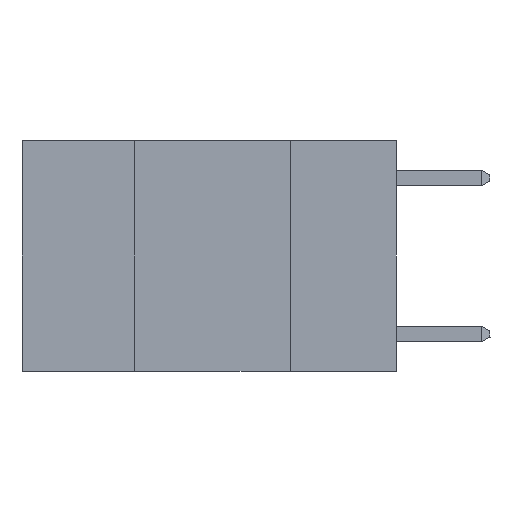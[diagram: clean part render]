
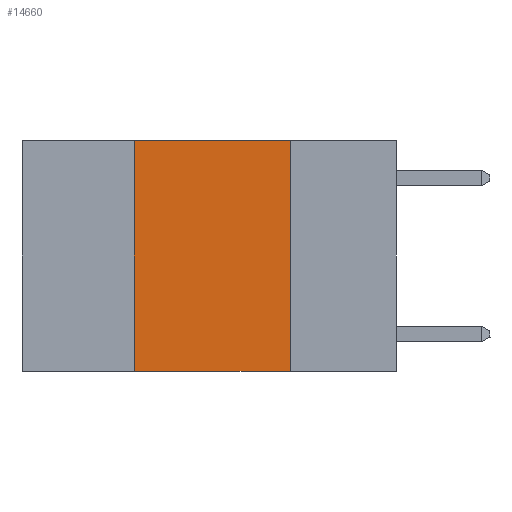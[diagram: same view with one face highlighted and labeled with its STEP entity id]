
A CAD part, left-side view. The second image highlights one B-rep face of the part: STEP entity #14660.
In plain terms, the highlighted planar face has unit normal (-1, 0, 0).
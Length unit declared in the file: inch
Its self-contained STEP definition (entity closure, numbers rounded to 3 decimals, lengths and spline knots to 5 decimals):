
#865 = EDGE_CURVE ( 'NONE', #9889, #1919, #4138, .T. ) ;
#1919 = VERTEX_POINT ( 'NONE', #10602 ) ;
#2404 = EDGE_LOOP ( 'NONE', ( #18171, #5483, #12597, #16038 ) ) ;
#4036 = DIRECTION ( 'NONE',  ( 0., 0., -1. ) ) ;
#4138 = LINE ( 'NONE', #13266, #10426 ) ;
#4831 = DIRECTION ( 'NONE',  ( 0., -1., 0. ) ) ;
#5483 = ORIENTED_EDGE ( 'NONE', *, *, #865, .F. ) ;
#5549 = DIRECTION ( 'NONE',  ( 0., 0., -1. ) ) ;
#6159 = EDGE_CURVE ( 'NONE', #1919, #14884, #16124, .T. ) ;
#6454 = VECTOR ( 'NONE', #4831, 39.37008 ) ;
#6555 = LINE ( 'NONE', #10590, #6454 ) ;
#7171 = FACE_OUTER_BOUND ( 'NONE', #2404, .T. ) ;
#7272 = PLANE ( 'NONE',  #15647 ) ;
#7776 = EDGE_CURVE ( 'NONE', #9317, #14884, #6555, .T. ) ;
#7943 = CARTESIAN_POINT ( 'NONE',  ( 0., 0.17, -0.37 ) ) ;
#9317 = VERTEX_POINT ( 'NONE', #15945 ) ;
#9889 = VERTEX_POINT ( 'NONE', #15029 ) ;
#10426 = VECTOR ( 'NONE', #14701, 39.37008 ) ;
#10590 = CARTESIAN_POINT ( 'NONE',  ( 0., 0.6, -0.37 ) ) ;
#10602 = CARTESIAN_POINT ( 'NONE',  ( 0., 0.17, 0. ) ) ;
#11338 = CARTESIAN_POINT ( 'NONE',  ( 0., 0.17, 0. ) ) ;
#12597 = ORIENTED_EDGE ( 'NONE', *, *, #18457, .F. ) ;
#13266 = CARTESIAN_POINT ( 'NONE',  ( 0., 0.6, 0. ) ) ;
#13400 = VECTOR ( 'NONE', #18390, 39.37008 ) ;
#14282 = DIRECTION ( 'NONE',  ( 1., 0., 0. ) ) ;
#14584 = VECTOR ( 'NONE', #4036, 39.37008 ) ;
#14660 = ADVANCED_FACE ( 'NONE', ( #7171 ), #7272, .F. ) ;
#14701 = DIRECTION ( 'NONE',  ( 0., -1., 0. ) ) ;
#14884 = VERTEX_POINT ( 'NONE', #7943 ) ;
#15029 = CARTESIAN_POINT ( 'NONE',  ( 0., 0.42, 0. ) ) ;
#15229 = LINE ( 'NONE', #15424, #13400 ) ;
#15424 = CARTESIAN_POINT ( 'NONE',  ( 0., 0.42, 0. ) ) ;
#15647 = AXIS2_PLACEMENT_3D ( 'NONE', #18928, #14282, #5549 ) ;
#15945 = CARTESIAN_POINT ( 'NONE',  ( 0., 0.42, -0.37 ) ) ;
#16038 = ORIENTED_EDGE ( 'NONE', *, *, #7776, .T. ) ;
#16124 = LINE ( 'NONE', #11338, #14584 ) ;
#18171 = ORIENTED_EDGE ( 'NONE', *, *, #6159, .F. ) ;
#18390 = DIRECTION ( 'NONE',  ( 0., 0., 1. ) ) ;
#18457 = EDGE_CURVE ( 'NONE', #9317, #9889, #15229, .T. ) ;
#18928 = CARTESIAN_POINT ( 'NONE',  ( 0., 0.6, 0. ) ) ;
